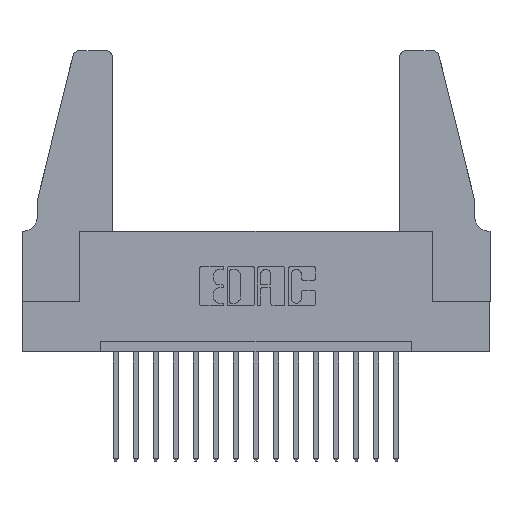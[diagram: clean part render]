
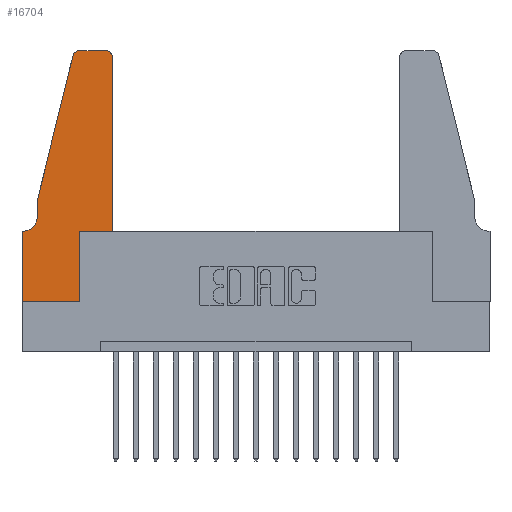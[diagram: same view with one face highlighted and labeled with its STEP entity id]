
A CAD part, top view. The second image highlights one B-rep face of the part: STEP entity #16704.
In plain terms, the highlighted planar face has unit normal (0, 0, 1).
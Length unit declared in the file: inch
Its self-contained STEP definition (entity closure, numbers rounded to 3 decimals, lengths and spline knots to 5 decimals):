
#122 = LINE ( 'NONE', #3927, #7179 ) ;
#133 = VERTEX_POINT ( 'NONE', #9832 ) ;
#228 = CARTESIAN_POINT ( 'NONE',  ( 0., 0., 0.37 ) ) ;
#392 = DIRECTION ( 'NONE',  ( -1., 0., 0. ) ) ;
#525 = ORIENTED_EDGE ( 'NONE', *, *, #11193, .T. ) ;
#527 = DIRECTION ( 'NONE',  ( -0.239, -0.971, 0. ) ) ;
#591 = LINE ( 'NONE', #9491, #14019 ) ;
#646 = AXIS2_PLACEMENT_3D ( 'NONE', #14502, #7825, #17099 ) ;
#732 = LINE ( 'NONE', #4975, #8613 ) ;
#803 = AXIS2_PLACEMENT_3D ( 'NONE', #6133, #16693, #2085 ) ;
#959 = ORIENTED_EDGE ( 'NONE', *, *, #10534, .T. ) ;
#1057 = EDGE_CURVE ( 'NONE', #14863, #8528, #4219, .T. ) ;
#1126 = VERTEX_POINT ( 'NONE', #8982 ) ;
#1229 = VECTOR ( 'NONE', #12006, 39.37008 ) ;
#1341 = VERTEX_POINT ( 'NONE', #5619 ) ;
#1687 = CARTESIAN_POINT ( 'NONE',  ( 0.0755, 0.35, 0.37 ) ) ;
#2077 = CIRCLE ( 'NONE', #4198, 0.07 ) ;
#2085 = DIRECTION ( 'NONE',  ( 1., 0., 0. ) ) ;
#2127 = VERTEX_POINT ( 'NONE', #5140 ) ;
#2204 = CARTESIAN_POINT ( 'NONE',  ( 0., 0., 0.37 ) ) ;
#2434 = DIRECTION ( 'NONE',  ( 0., 0., 1. ) ) ;
#2657 = CIRCLE ( 'NONE', #803, 0.03 ) ;
#2708 = DIRECTION ( 'NONE',  ( 1., 0., 0. ) ) ;
#2861 = ORIENTED_EDGE ( 'NONE', *, *, #15555, .T. ) ;
#2900 = VECTOR ( 'NONE', #10885, 39.37008 ) ;
#3467 = VERTEX_POINT ( 'NONE', #14555 ) ;
#3854 = ORIENTED_EDGE ( 'NONE', *, *, #8721, .T. ) ;
#3927 = CARTESIAN_POINT ( 'NONE',  ( 0.4505, 0.35, 0.37 ) ) ;
#4100 = DIRECTION ( 'NONE',  ( 1., 0., 0. ) ) ;
#4198 = AXIS2_PLACEMENT_3D ( 'NONE', #16375, #8353, #392 ) ;
#4219 = LINE ( 'NONE', #9154, #9173 ) ;
#4302 = VERTEX_POINT ( 'NONE', #16495 ) ;
#4342 = LINE ( 'NONE', #11925, #2900 ) ;
#4975 = CARTESIAN_POINT ( 'NONE',  ( 0.4505, 0.35, 0.37 ) ) ;
#5140 = CARTESIAN_POINT ( 'NONE',  ( 0.4505, 0.35, 0.37 ) ) ;
#5168 = DIRECTION ( 'NONE',  ( -1., 0., 0. ) ) ;
#5235 = DIRECTION ( 'NONE',  ( 0., 1., 0. ) ) ;
#5279 = ORIENTED_EDGE ( 'NONE', *, *, #1057, .T. ) ;
#5309 = AXIS2_PLACEMENT_3D ( 'NONE', #7762, #2434, #11828 ) ;
#5619 = CARTESIAN_POINT ( 'NONE',  ( 0.4505, 1.22, 0.37 ) ) ;
#5683 = DIRECTION ( 'NONE',  ( 0., -1., 0. ) ) ;
#6002 = EDGE_CURVE ( 'NONE', #8528, #4302, #16598, .T. ) ;
#6133 = CARTESIAN_POINT ( 'NONE',  ( 0.4205, 1.22, 0.37 ) ) ;
#6316 = CARTESIAN_POINT ( 'NONE',  ( 0.2865, 0., 0.37 ) ) ;
#6960 = ORIENTED_EDGE ( 'NONE', *, *, #8267, .T. ) ;
#7135 = EDGE_LOOP ( 'NONE', ( #5279, #14553, #525, #3854, #2861, #11046, #10285, #15750, #6960, #8300, #12097, #959 ) ) ;
#7179 = VECTOR ( 'NONE', #2708, 39.37008 ) ;
#7762 = CARTESIAN_POINT ( 'NONE',  ( 0., 0.35, 0.37 ) ) ;
#7825 = DIRECTION ( 'NONE',  ( 0., 0., 1. ) ) ;
#8267 = EDGE_CURVE ( 'NONE', #16846, #133, #12585, .T. ) ;
#8300 = ORIENTED_EDGE ( 'NONE', *, *, #11391, .T. ) ;
#8353 = DIRECTION ( 'NONE',  ( 0., 0., -1. ) ) ;
#8528 = VERTEX_POINT ( 'NONE', #13903 ) ;
#8613 = VECTOR ( 'NONE', #16703, 39.37008 ) ;
#8629 = VECTOR ( 'NONE', #4100, 39.37008 ) ;
#8721 = EDGE_CURVE ( 'NONE', #1126, #3467, #591, .T. ) ;
#8871 = LINE ( 'NONE', #1687, #1229 ) ;
#8982 = CARTESIAN_POINT ( 'NONE',  ( 0.0755, 0.5, 0.37 ) ) ;
#9132 = CARTESIAN_POINT ( 'NONE',  ( 0.0055, 0.35, 0.37 ) ) ;
#9154 = CARTESIAN_POINT ( 'NONE',  ( 0.2605, 1.25, 0.37 ) ) ;
#9173 = VECTOR ( 'NONE', #5168, 39.37008 ) ;
#9491 = CARTESIAN_POINT ( 'NONE',  ( 0.0755, 0.5, 0.37 ) ) ;
#9826 = CARTESIAN_POINT ( 'NONE',  ( 0.0755, 0.5, 0.37 ) ) ;
#9832 = CARTESIAN_POINT ( 'NONE',  ( 0.2865, 0.35, 0.37 ) ) ;
#9864 = LINE ( 'NONE', #9826, #11102 ) ;
#9985 = VERTEX_POINT ( 'NONE', #9132 ) ;
#10285 = ORIENTED_EDGE ( 'NONE', *, *, #15493, .T. ) ;
#10354 = PLANE ( 'NONE',  #5309 ) ;
#10534 = EDGE_CURVE ( 'NONE', #1341, #14863, #2657, .T. ) ;
#10687 = CARTESIAN_POINT ( 'NONE',  ( 0.4205, 1.25, 0.37 ) ) ;
#10885 = DIRECTION ( 'NONE',  ( 0., -1., 0. ) ) ;
#11046 = ORIENTED_EDGE ( 'NONE', *, *, #16023, .T. ) ;
#11102 = VECTOR ( 'NONE', #527, 39.37008 ) ;
#11193 = EDGE_CURVE ( 'NONE', #4302, #1126, #9864, .T. ) ;
#11391 = EDGE_CURVE ( 'NONE', #133, #2127, #122, .T. ) ;
#11828 = DIRECTION ( 'NONE',  ( 1., 0., 0. ) ) ;
#11925 = CARTESIAN_POINT ( 'NONE',  ( 0., 0., 0.37 ) ) ;
#12006 = DIRECTION ( 'NONE',  ( -1., 0., 0. ) ) ;
#12097 = ORIENTED_EDGE ( 'NONE', *, *, #16886, .T. ) ;
#12585 = LINE ( 'NONE', #13419, #15693 ) ;
#13419 = CARTESIAN_POINT ( 'NONE',  ( 0.2865, 0.35, 0.37 ) ) ;
#13903 = CARTESIAN_POINT ( 'NONE',  ( 0.284, 1.25, 0.37 ) ) ;
#14019 = VECTOR ( 'NONE', #5683, 39.37008 ) ;
#14502 = CARTESIAN_POINT ( 'NONE',  ( 0.284, 1.22, 0.37 ) ) ;
#14553 = ORIENTED_EDGE ( 'NONE', *, *, #6002, .T. ) ;
#14555 = CARTESIAN_POINT ( 'NONE',  ( 0.0755, 0.42, 0.37 ) ) ;
#14588 = VERTEX_POINT ( 'NONE', #16872 ) ;
#14863 = VERTEX_POINT ( 'NONE', #10687 ) ;
#15493 = EDGE_CURVE ( 'NONE', #14588, #16550, #4342, .T. ) ;
#15555 = EDGE_CURVE ( 'NONE', #3467, #9985, #2077, .T. ) ;
#15693 = VECTOR ( 'NONE', #5235, 39.37008 ) ;
#15750 = ORIENTED_EDGE ( 'NONE', *, *, #16762, .T. ) ;
#16023 = EDGE_CURVE ( 'NONE', #9985, #14588, #8871, .T. ) ;
#16258 = FACE_OUTER_BOUND ( 'NONE', #7135, .T. ) ;
#16375 = CARTESIAN_POINT ( 'NONE',  ( 0.0055, 0.42, 0.37 ) ) ;
#16495 = CARTESIAN_POINT ( 'NONE',  ( 0.25487, 1.22718, 0.37 ) ) ;
#16550 = VERTEX_POINT ( 'NONE', #2204 ) ;
#16598 = CIRCLE ( 'NONE', #646, 0.03 ) ;
#16693 = DIRECTION ( 'NONE',  ( 0., 0., 1. ) ) ;
#16703 = DIRECTION ( 'NONE',  ( 0., 1., 0. ) ) ;
#16704 = ADVANCED_FACE ( 'NONE', ( #16258 ), #10354, .T. ) ;
#16762 = EDGE_CURVE ( 'NONE', #16550, #16846, #16873, .T. ) ;
#16846 = VERTEX_POINT ( 'NONE', #6316 ) ;
#16872 = CARTESIAN_POINT ( 'NONE',  ( 0., 0.35, 0.37 ) ) ;
#16873 = LINE ( 'NONE', #228, #8629 ) ;
#16886 = EDGE_CURVE ( 'NONE', #2127, #1341, #732, .T. ) ;
#17099 = DIRECTION ( 'NONE',  ( 1., 0., 0. ) ) ;
